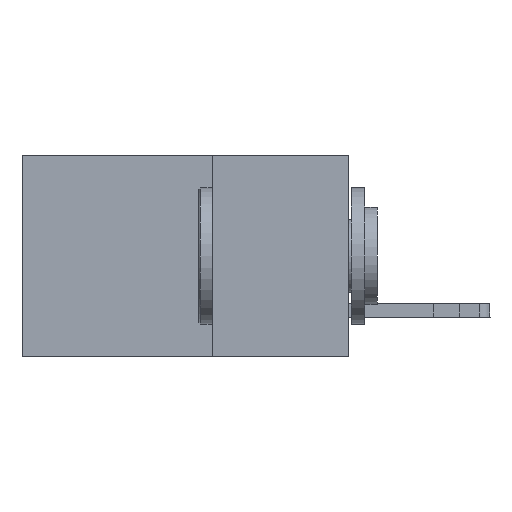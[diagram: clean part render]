
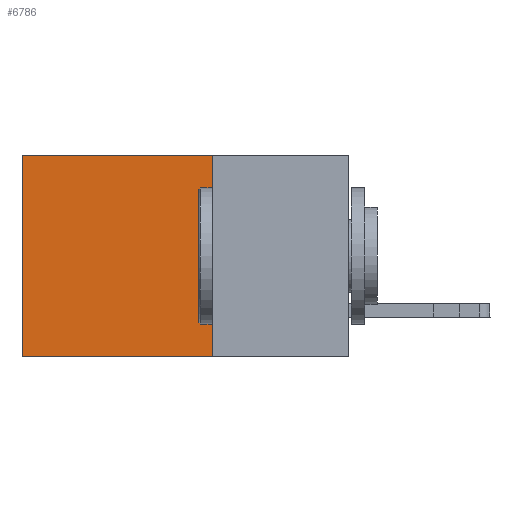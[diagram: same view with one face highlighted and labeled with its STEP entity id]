
A CAD part, left-side view. The second image highlights one B-rep face of the part: STEP entity #6786.
In plain terms, the highlighted planar face has unit normal (-1, 0, 0).
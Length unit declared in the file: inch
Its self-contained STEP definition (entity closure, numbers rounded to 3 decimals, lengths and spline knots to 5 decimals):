
#606 = CARTESIAN_POINT ( 'NONE',  ( 0.298, 0.25, 0. ) ) ;
#982 = LINE ( 'NONE', #21433, #13137 ) ;
#1491 = ORIENTED_EDGE ( 'NONE', *, *, #11036, .T. ) ;
#1711 = CARTESIAN_POINT ( 'NONE',  ( 0.298, 0.6, 0. ) ) ;
#2025 = EDGE_CURVE ( 'NONE', #13094, #14477, #22265, .T. ) ;
#2542 = DIRECTION ( 'NONE',  ( 0., 0., -1. ) ) ;
#2791 = CARTESIAN_POINT ( 'NONE',  ( 0.298, 0.25, -0.37 ) ) ;
#4371 = ORIENTED_EDGE ( 'NONE', *, *, #21690, .T. ) ;
#4457 = AXIS2_PLACEMENT_3D ( 'NONE', #606, #6917, #2542 ) ;
#4474 = PLANE ( 'NONE',  #4457 ) ;
#4991 = FACE_OUTER_BOUND ( 'NONE', #23409, .T. ) ;
#5247 = CARTESIAN_POINT ( 'NONE',  ( 0.298, 0.25, -0.37 ) ) ;
#5718 = VECTOR ( 'NONE', #15273, 39.37008 ) ;
#6786 = ADVANCED_FACE ( 'NONE', ( #4991 ), #4474, .F. ) ;
#6917 = DIRECTION ( 'NONE',  ( 1., 0., 0. ) ) ;
#7425 = DIRECTION ( 'NONE',  ( 0., 1., 0. ) ) ;
#7530 = ORIENTED_EDGE ( 'NONE', *, *, #23045, .F. ) ;
#7862 = CARTESIAN_POINT ( 'NONE',  ( 0.298, 0.6, -0.37 ) ) ;
#9280 = CARTESIAN_POINT ( 'NONE',  ( 0.298, 0.6, 0. ) ) ;
#10328 = VECTOR ( 'NONE', #18196, 39.37008 ) ;
#11036 = EDGE_CURVE ( 'NONE', #18866, #24758, #18192, .T. ) ;
#11186 = LINE ( 'NONE', #9280, #5718 ) ;
#12527 = VECTOR ( 'NONE', #7425, 39.37008 ) ;
#13094 = VERTEX_POINT ( 'NONE', #2791 ) ;
#13137 = VECTOR ( 'NONE', #16952, 39.37008 ) ;
#14477 = VERTEX_POINT ( 'NONE', #7862 ) ;
#15273 = DIRECTION ( 'NONE',  ( 0., 0., -1. ) ) ;
#15330 = CARTESIAN_POINT ( 'NONE',  ( 0.298, 0.25, 0. ) ) ;
#16952 = DIRECTION ( 'NONE',  ( 0., 0., -1. ) ) ;
#18192 = LINE ( 'NONE', #21842, #12527 ) ;
#18196 = DIRECTION ( 'NONE',  ( 0., 1., 0. ) ) ;
#18866 = VERTEX_POINT ( 'NONE', #15330 ) ;
#21433 = CARTESIAN_POINT ( 'NONE',  ( 0.298, 0.25, 0. ) ) ;
#21690 = EDGE_CURVE ( 'NONE', #24758, #14477, #11186, .T. ) ;
#21842 = CARTESIAN_POINT ( 'NONE',  ( 0.298, 0.25, 0. ) ) ;
#22265 = LINE ( 'NONE', #5247, #10328 ) ;
#23045 = EDGE_CURVE ( 'NONE', #18866, #13094, #982, .T. ) ;
#23409 = EDGE_LOOP ( 'NONE', ( #4371, #25603, #7530, #1491 ) ) ;
#24758 = VERTEX_POINT ( 'NONE', #1711 ) ;
#25603 = ORIENTED_EDGE ( 'NONE', *, *, #2025, .F. ) ;
